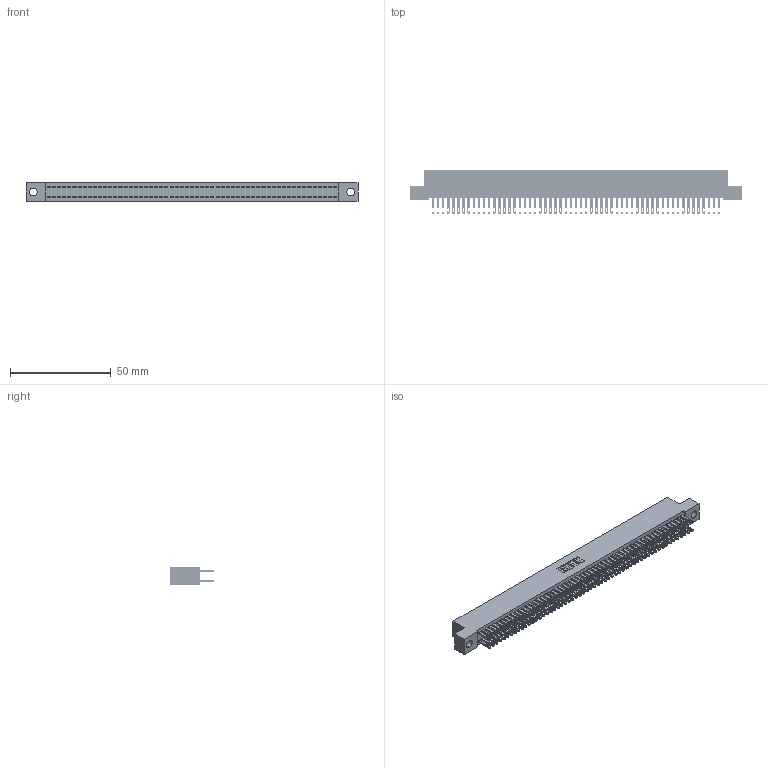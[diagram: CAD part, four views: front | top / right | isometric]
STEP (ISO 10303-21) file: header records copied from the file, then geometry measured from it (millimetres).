
FILE_DESCRIPTION (( 'STEP AP203' ), '1' );
FILE_NAME ('342-114-500-204.STEP', '2019-10-04T21:19:23', ( '' ), ( '' ), 'SwSTEP 2.0', 'SolidWorks 2016', '' );
FILE_SCHEMA (( 'CONFIG_CONTROL_DESIGN' ));
Length unit declared in the file: inch
Products named in the file (3): 342 Part_.156 TH; 345-292-001_345-293-100; 342-114-500-204
Assembly tree (115 placements, depth 2):
  342-114-500-204
    342 Part_.156 TH
    345-292-001_345-293-100  x114
Bounding box: 165.1 x 21.85 x 9.4 mm (x, y, z)
Volume: 15166.5 mm3; surface area: 25972.6 mm2
Topology: 115 solids, 115 shells, 5582 faces, 17057 edges, 11370 vertices
Faces by surface type: plane 3486, cylinder 2096
Entity records: 34531 total; most frequent: CARTESIAN_POINT 5702, ORIENTED_EDGE 5638, DIRECTION 4847, EDGE_CURVE 2819, LINE 2687, VECTOR 2687, VERTEX_POINT 1878, AXIS2_PLACEMENT_3D 1080
